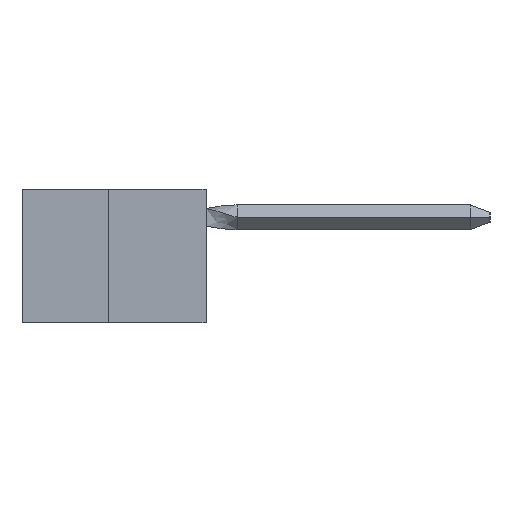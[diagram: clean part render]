
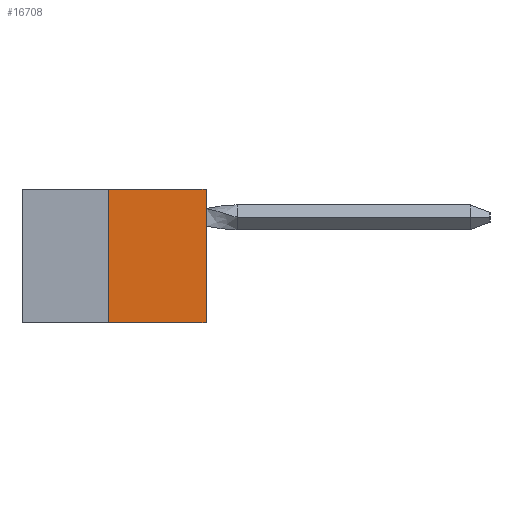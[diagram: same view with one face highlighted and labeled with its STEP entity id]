
A CAD part, left-side view. The second image highlights one B-rep face of the part: STEP entity #16708.
In plain terms, the highlighted planar face has unit normal (-1, 0, 0).
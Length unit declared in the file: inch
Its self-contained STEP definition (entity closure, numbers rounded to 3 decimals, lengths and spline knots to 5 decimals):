
#745 = CARTESIAN_POINT ( 'NONE',  ( 0., 0.473, -0.343 ) ) ;
#832 = AXIS2_PLACEMENT_3D ( 'NONE', #16296, #26231, #16094 ) ;
#1349 = LINE ( 'NONE', #16430, #27549 ) ;
#2843 = CARTESIAN_POINT ( 'NONE',  ( 0., 0.473, 0. ) ) ;
#2954 = DIRECTION ( 'NONE',  ( 0., -1., 0. ) ) ;
#3401 = PLANE ( 'NONE',  #832 ) ;
#6375 = VECTOR ( 'NONE', #2954, 39.37008 ) ;
#7693 = VECTOR ( 'NONE', #11534, 39.37008 ) ;
#7835 = EDGE_CURVE ( 'NONE', #8211, #14687, #1349, .T. ) ;
#7906 = LINE ( 'NONE', #21741, #16669 ) ;
#8211 = VERTEX_POINT ( 'NONE', #20561 ) ;
#8499 = LINE ( 'NONE', #745, #7693 ) ;
#8527 = DIRECTION ( 'NONE',  ( 0., 0., 1. ) ) ;
#10357 = FACE_OUTER_BOUND ( 'NONE', #23030, .T. ) ;
#11534 = DIRECTION ( 'NONE',  ( 0., -1., 0. ) ) ;
#13485 = CARTESIAN_POINT ( 'NONE',  ( 0., 0.25, 0. ) ) ;
#14687 = VERTEX_POINT ( 'NONE', #18183 ) ;
#14765 = ORIENTED_EDGE ( 'NONE', *, *, #16551, .F. ) ;
#15114 = ORIENTED_EDGE ( 'NONE', *, *, #17711, .T. ) ;
#16094 = DIRECTION ( 'NONE',  ( 0., 0., -1. ) ) ;
#16296 = CARTESIAN_POINT ( 'NONE',  ( 0., 0.473, 0. ) ) ;
#16430 = CARTESIAN_POINT ( 'NONE',  ( 0., 0., 0. ) ) ;
#16551 = EDGE_CURVE ( 'NONE', #21175, #14687, #32117, .T. ) ;
#16669 = VECTOR ( 'NONE', #21987, 39.37008 ) ;
#16708 = ADVANCED_FACE ( 'NONE', ( #10357 ), #3401, .F. ) ;
#17057 = VERTEX_POINT ( 'NONE', #22805 ) ;
#17711 = EDGE_CURVE ( 'NONE', #17057, #8211, #8499, .T. ) ;
#18183 = CARTESIAN_POINT ( 'NONE',  ( 0., 0., 0. ) ) ;
#20561 = CARTESIAN_POINT ( 'NONE',  ( 0., 0., -0.343 ) ) ;
#21175 = VERTEX_POINT ( 'NONE', #13485 ) ;
#21741 = CARTESIAN_POINT ( 'NONE',  ( 0., 0.25, 0. ) ) ;
#21987 = DIRECTION ( 'NONE',  ( 0., 0., 1. ) ) ;
#22805 = CARTESIAN_POINT ( 'NONE',  ( 0., 0.25, -0.343 ) ) ;
#23030 = EDGE_LOOP ( 'NONE', ( #14765, #26525, #15114, #23739 ) ) ;
#23738 = EDGE_CURVE ( 'NONE', #17057, #21175, #7906, .T. ) ;
#23739 = ORIENTED_EDGE ( 'NONE', *, *, #7835, .T. ) ;
#26231 = DIRECTION ( 'NONE',  ( 1., 0., 0. ) ) ;
#26525 = ORIENTED_EDGE ( 'NONE', *, *, #23738, .F. ) ;
#27549 = VECTOR ( 'NONE', #8527, 39.37008 ) ;
#32117 = LINE ( 'NONE', #2843, #6375 ) ;
